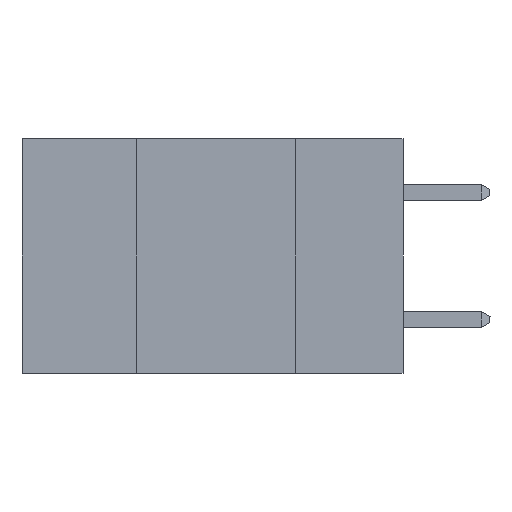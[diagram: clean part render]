
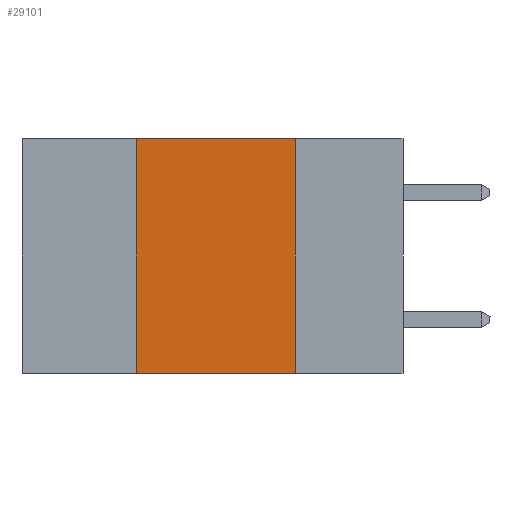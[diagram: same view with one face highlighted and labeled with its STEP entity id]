
A CAD part, left-side view. The second image highlights one B-rep face of the part: STEP entity #29101.
In plain terms, the highlighted planar face has unit normal (-1, 0, 0).
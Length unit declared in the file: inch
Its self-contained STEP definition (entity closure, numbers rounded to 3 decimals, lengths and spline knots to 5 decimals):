
#233 = DIRECTION ( 'NONE',  ( 0., 0., -1. ) ) ;
#617 = CARTESIAN_POINT ( 'NONE',  ( 0., 0.17, -0.37 ) ) ;
#2246 = LINE ( 'NONE', #38542, #28116 ) ;
#2989 = DIRECTION ( 'NONE',  ( 0., 0., 1. ) ) ;
#3206 = CARTESIAN_POINT ( 'NONE',  ( 0., 0.17, 0. ) ) ;
#7072 = EDGE_CURVE ( 'NONE', #23825, #29662, #36596, .T. ) ;
#8421 = LINE ( 'NONE', #21586, #13943 ) ;
#9913 = CARTESIAN_POINT ( 'NONE',  ( 0., 0.42, 0. ) ) ;
#10606 = FACE_OUTER_BOUND ( 'NONE', #33674, .T. ) ;
#13257 = ORIENTED_EDGE ( 'NONE', *, *, #24535, .T. ) ;
#13943 = VECTOR ( 'NONE', #41032, 39.37008 ) ;
#15788 = ORIENTED_EDGE ( 'NONE', *, *, #34196, .F. ) ;
#16868 = PLANE ( 'NONE',  #25223 ) ;
#17524 = VECTOR ( 'NONE', #29901, 39.37008 ) ;
#19176 = VECTOR ( 'NONE', #2989, 39.37008 ) ;
#19673 = DIRECTION ( 'NONE',  ( 1., 0., 0. ) ) ;
#21586 = CARTESIAN_POINT ( 'NONE',  ( 0., 0.6, -0.37 ) ) ;
#23825 = VERTEX_POINT ( 'NONE', #33481 ) ;
#24535 = EDGE_CURVE ( 'NONE', #29017, #41322, #8421, .T. ) ;
#25223 = AXIS2_PLACEMENT_3D ( 'NONE', #32860, #19673, #233 ) ;
#25756 = CARTESIAN_POINT ( 'NONE',  ( 0., 0.42, -0.37 ) ) ;
#26016 = DIRECTION ( 'NONE',  ( 0., 0., -1. ) ) ;
#26468 = CARTESIAN_POINT ( 'NONE',  ( 0., 0.6, 0. ) ) ;
#28116 = VECTOR ( 'NONE', #26016, 39.37008 ) ;
#29017 = VERTEX_POINT ( 'NONE', #25756 ) ;
#29101 = ADVANCED_FACE ( 'NONE', ( #10606 ), #16868, .F. ) ;
#29662 = VERTEX_POINT ( 'NONE', #3206 ) ;
#29901 = DIRECTION ( 'NONE',  ( 0., -1., 0. ) ) ;
#32860 = CARTESIAN_POINT ( 'NONE',  ( 0., 0.6, 0. ) ) ;
#33309 = EDGE_CURVE ( 'NONE', #29662, #41322, #2246, .T. ) ;
#33481 = CARTESIAN_POINT ( 'NONE',  ( 0., 0.42, 0. ) ) ;
#33674 = EDGE_LOOP ( 'NONE', ( #34344, #39125, #15788, #13257 ) ) ;
#34196 = EDGE_CURVE ( 'NONE', #29017, #23825, #40279, .T. ) ;
#34344 = ORIENTED_EDGE ( 'NONE', *, *, #33309, .F. ) ;
#36596 = LINE ( 'NONE', #26468, #17524 ) ;
#38542 = CARTESIAN_POINT ( 'NONE',  ( 0., 0.17, 0. ) ) ;
#39125 = ORIENTED_EDGE ( 'NONE', *, *, #7072, .F. ) ;
#40279 = LINE ( 'NONE', #9913, #19176 ) ;
#41032 = DIRECTION ( 'NONE',  ( 0., -1., 0. ) ) ;
#41322 = VERTEX_POINT ( 'NONE', #617 ) ;
